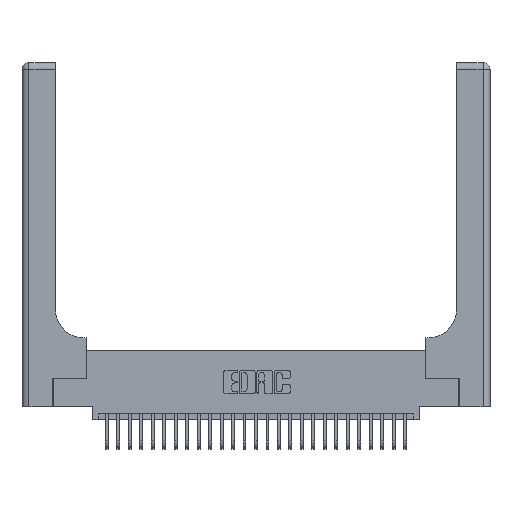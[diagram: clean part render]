
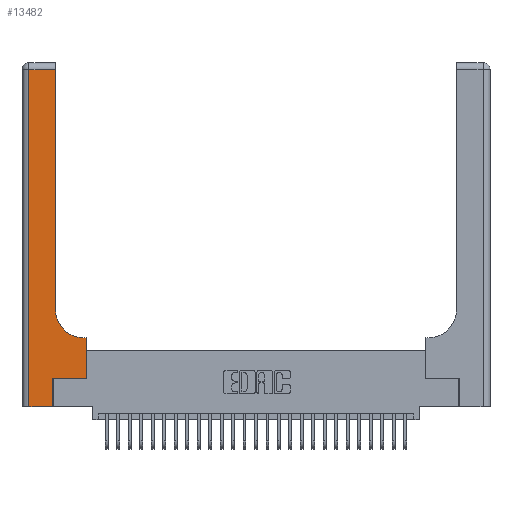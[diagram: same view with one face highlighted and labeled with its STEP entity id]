
A CAD part, top view. The second image highlights one B-rep face of the part: STEP entity #13482.
In plain terms, the highlighted planar face has unit normal (0, 0, 1).
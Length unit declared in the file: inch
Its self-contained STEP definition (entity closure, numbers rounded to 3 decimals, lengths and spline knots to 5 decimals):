
#237 = EDGE_CURVE ( 'NONE', #2752, #17183, #22455, .T. ) ;
#1459 = ORIENTED_EDGE ( 'NONE', *, *, #27019, .T. ) ;
#1781 = CARTESIAN_POINT ( 'NONE',  ( 0.06, 3., 0.37 ) ) ;
#2752 = VERTEX_POINT ( 'NONE', #23680 ) ;
#3194 = VERTEX_POINT ( 'NONE', #27903 ) ;
#4206 = VERTEX_POINT ( 'NONE', #18315 ) ;
#5823 = VERTEX_POINT ( 'NONE', #14317 ) ;
#5952 = ORIENTED_EDGE ( 'NONE', *, *, #9147, .T. ) ;
#6055 = LINE ( 'NONE', #24724, #17738 ) ;
#6247 = CARTESIAN_POINT ( 'NONE',  ( 0.269, 0., 0.37 ) ) ;
#7192 = PLANE ( 'NONE',  #16944 ) ;
#7713 = DIRECTION ( 'NONE',  ( -1., 0., 0. ) ) ;
#7735 = DIRECTION ( 'NONE',  ( 1., 0., 0. ) ) ;
#7835 = DIRECTION ( 'NONE',  ( 0., 0., -1. ) ) ;
#7938 = CARTESIAN_POINT ( 'NONE',  ( 0.5415, 0.85, 0.37 ) ) ;
#8218 = CARTESIAN_POINT ( 'NONE',  ( 0.2915, 2.94, 0.37 ) ) ;
#9147 = EDGE_CURVE ( 'NONE', #3194, #17069, #24837, .T. ) ;
#9563 = DIRECTION ( 'NONE',  ( -1., 0., 0. ) ) ;
#9890 = VERTEX_POINT ( 'NONE', #22563 ) ;
#10078 = CARTESIAN_POINT ( 'NONE',  ( 0.2915, 0.6, 0.37 ) ) ;
#11435 = CARTESIAN_POINT ( 'NONE',  ( 0.5585, 0.25, 0.37 ) ) ;
#11597 = CARTESIAN_POINT ( 'NONE',  ( 0.5585, 0.6, 0.37 ) ) ;
#11658 = EDGE_LOOP ( 'NONE', ( #25528, #1459, #15449, #27699, #23009, #5952, #12231, #24457, #19818 ) ) ;
#11866 = EDGE_CURVE ( 'NONE', #25038, #2752, #13977, .T. ) ;
#12231 = ORIENTED_EDGE ( 'NONE', *, *, #19007, .T. ) ;
#12824 = EDGE_CURVE ( 'NONE', #4206, #5823, #26897, .T. ) ;
#13482 = ADVANCED_FACE ( 'NONE', ( #28989 ), #7192, .F. ) ;
#13743 = DIRECTION ( 'NONE',  ( 0., 1., 0. ) ) ;
#13852 = EDGE_CURVE ( 'NONE', #5823, #9890, #15659, .T. ) ;
#13977 = LINE ( 'NONE', #10078, #14717 ) ;
#14214 = VECTOR ( 'NONE', #26237, 39.37008 ) ;
#14317 = CARTESIAN_POINT ( 'NONE',  ( 0.06, 0., 0.37 ) ) ;
#14334 = AXIS2_PLACEMENT_3D ( 'NONE', #7938, #7835, #7735 ) ;
#14658 = VERTEX_POINT ( 'NONE', #8218 ) ;
#14717 = VECTOR ( 'NONE', #7713, 39.37008 ) ;
#15073 = CARTESIAN_POINT ( 'NONE',  ( 0.5585, 0.25, 0.37 ) ) ;
#15371 = DIRECTION ( 'NONE',  ( 1., 0., 0. ) ) ;
#15449 = ORIENTED_EDGE ( 'NONE', *, *, #12824, .T. ) ;
#15520 = VECTOR ( 'NONE', #23646, 39.37008 ) ;
#15659 = LINE ( 'NONE', #26137, #14214 ) ;
#16317 = LINE ( 'NONE', #11435, #27823 ) ;
#16555 = LINE ( 'NONE', #6247, #21943 ) ;
#16944 = AXIS2_PLACEMENT_3D ( 'NONE', #30163, #23352, #9563 ) ;
#17069 = VERTEX_POINT ( 'NONE', #15073 ) ;
#17183 = VERTEX_POINT ( 'NONE', #17814 ) ;
#17738 = VECTOR ( 'NONE', #18010, 39.37008 ) ;
#17814 = CARTESIAN_POINT ( 'NONE',  ( 0.2915, 0.85, 0.37 ) ) ;
#18010 = DIRECTION ( 'NONE',  ( 0., 1., 0. ) ) ;
#18315 = CARTESIAN_POINT ( 'NONE',  ( 0.06, 2.94, 0.37 ) ) ;
#18770 = VECTOR ( 'NONE', #15371, 39.37008 ) ;
#19007 = EDGE_CURVE ( 'NONE', #17069, #25038, #16317, .T. ) ;
#19404 = EDGE_CURVE ( 'NONE', #17183, #14658, #6055, .T. ) ;
#19818 = ORIENTED_EDGE ( 'NONE', *, *, #237, .T. ) ;
#19935 = CARTESIAN_POINT ( 'NONE',  ( 0.269, 0.25, 0.37 ) ) ;
#20066 = VECTOR ( 'NONE', #29704, 39.37008 ) ;
#20195 = DIRECTION ( 'NONE',  ( 0., 1., 0. ) ) ;
#21348 = CARTESIAN_POINT ( 'NONE',  ( 0., 2.94, 0.37 ) ) ;
#21767 = EDGE_CURVE ( 'NONE', #9890, #3194, #16555, .T. ) ;
#21943 = VECTOR ( 'NONE', #20195, 39.37008 ) ;
#22455 = CIRCLE ( 'NONE', #14334, 0.25 ) ;
#22563 = CARTESIAN_POINT ( 'NONE',  ( 0.269, 0., 0.37 ) ) ;
#23009 = ORIENTED_EDGE ( 'NONE', *, *, #21767, .T. ) ;
#23352 = DIRECTION ( 'NONE',  ( 0., 0., -1. ) ) ;
#23646 = DIRECTION ( 'NONE',  ( -1., 0., 0. ) ) ;
#23680 = CARTESIAN_POINT ( 'NONE',  ( 0.5415, 0.6, 0.37 ) ) ;
#24457 = ORIENTED_EDGE ( 'NONE', *, *, #11866, .T. ) ;
#24724 = CARTESIAN_POINT ( 'NONE',  ( 0.2915, 3., 0.37 ) ) ;
#24837 = LINE ( 'NONE', #19935, #18770 ) ;
#25038 = VERTEX_POINT ( 'NONE', #11597 ) ;
#25528 = ORIENTED_EDGE ( 'NONE', *, *, #19404, .T. ) ;
#26137 = CARTESIAN_POINT ( 'NONE',  ( 0., 0., 0.37 ) ) ;
#26237 = DIRECTION ( 'NONE',  ( 1., 0., 0. ) ) ;
#26897 = LINE ( 'NONE', #1781, #20066 ) ;
#27019 = EDGE_CURVE ( 'NONE', #14658, #4206, #27778, .T. ) ;
#27699 = ORIENTED_EDGE ( 'NONE', *, *, #13852, .T. ) ;
#27778 = LINE ( 'NONE', #21348, #15520 ) ;
#27823 = VECTOR ( 'NONE', #13743, 39.37008 ) ;
#27903 = CARTESIAN_POINT ( 'NONE',  ( 0.269, 0.25, 0.37 ) ) ;
#28989 = FACE_OUTER_BOUND ( 'NONE', #11658, .T. ) ;
#29704 = DIRECTION ( 'NONE',  ( 0., -1., 0. ) ) ;
#30163 = CARTESIAN_POINT ( 'NONE',  ( 0., 3., 0.37 ) ) ;
